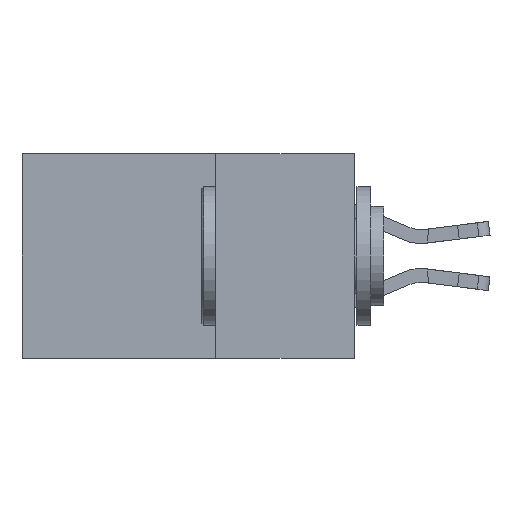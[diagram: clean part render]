
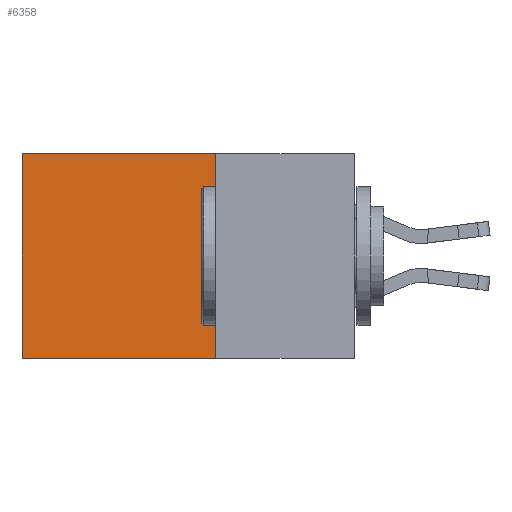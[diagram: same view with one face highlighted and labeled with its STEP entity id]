
A CAD part, left-side view. The second image highlights one B-rep face of the part: STEP entity #6358.
In plain terms, the highlighted planar face has unit normal (-1, 0, 0).
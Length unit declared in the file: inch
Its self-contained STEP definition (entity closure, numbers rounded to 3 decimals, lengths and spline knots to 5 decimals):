
#101 = LINE ( 'NONE', #17166, #5047 ) ;
#1664 = VECTOR ( 'NONE', #15389, 39.37008 ) ;
#1734 = VERTEX_POINT ( 'NONE', #1773 ) ;
#1773 = CARTESIAN_POINT ( 'NONE',  ( 0.298, 0.6, 0. ) ) ;
#2324 = EDGE_CURVE ( 'NONE', #1734, #3063, #101, .T. ) ;
#2328 = LINE ( 'NONE', #13277, #1664 ) ;
#3034 = VECTOR ( 'NONE', #15532, 39.37008 ) ;
#3063 = VERTEX_POINT ( 'NONE', #16732 ) ;
#3179 = ORIENTED_EDGE ( 'NONE', *, *, #2324, .T. ) ;
#3963 = EDGE_CURVE ( 'NONE', #17649, #3063, #8640, .T. ) ;
#4209 = CARTESIAN_POINT ( 'NONE',  ( 0.298, 0.25, 0. ) ) ;
#5047 = VECTOR ( 'NONE', #17201, 39.37008 ) ;
#6358 = ADVANCED_FACE ( 'NONE', ( #7459 ), #25138, .F. ) ;
#7459 = FACE_OUTER_BOUND ( 'NONE', #21451, .T. ) ;
#7604 = AXIS2_PLACEMENT_3D ( 'NONE', #24781, #22702, #22468 ) ;
#8640 = LINE ( 'NONE', #18347, #3034 ) ;
#8974 = CARTESIAN_POINT ( 'NONE',  ( 0.298, 0.25, -0.37 ) ) ;
#13277 = CARTESIAN_POINT ( 'NONE',  ( 0.298, 0.25, 0. ) ) ;
#13400 = DIRECTION ( 'NONE',  ( 0., 1., 0. ) ) ;
#14875 = EDGE_CURVE ( 'NONE', #24538, #1734, #20680, .T. ) ;
#15134 = VECTOR ( 'NONE', #13400, 39.37008 ) ;
#15389 = DIRECTION ( 'NONE',  ( 0., 0., -1. ) ) ;
#15532 = DIRECTION ( 'NONE',  ( 0., 1., 0. ) ) ;
#16732 = CARTESIAN_POINT ( 'NONE',  ( 0.298, 0.6, -0.37 ) ) ;
#17166 = CARTESIAN_POINT ( 'NONE',  ( 0.298, 0.6, 0. ) ) ;
#17201 = DIRECTION ( 'NONE',  ( 0., 0., -1. ) ) ;
#17649 = VERTEX_POINT ( 'NONE', #8974 ) ;
#18010 = ORIENTED_EDGE ( 'NONE', *, *, #18244, .F. ) ;
#18244 = EDGE_CURVE ( 'NONE', #24538, #17649, #2328, .T. ) ;
#18347 = CARTESIAN_POINT ( 'NONE',  ( 0.298, 0.25, -0.37 ) ) ;
#20680 = LINE ( 'NONE', #25838, #15134 ) ;
#21451 = EDGE_LOOP ( 'NONE', ( #3179, #27004, #18010, #24605 ) ) ;
#22468 = DIRECTION ( 'NONE',  ( 0., 0., -1. ) ) ;
#22702 = DIRECTION ( 'NONE',  ( 1., 0., 0. ) ) ;
#24538 = VERTEX_POINT ( 'NONE', #4209 ) ;
#24605 = ORIENTED_EDGE ( 'NONE', *, *, #14875, .T. ) ;
#24781 = CARTESIAN_POINT ( 'NONE',  ( 0.298, 0.25, 0. ) ) ;
#25138 = PLANE ( 'NONE',  #7604 ) ;
#25838 = CARTESIAN_POINT ( 'NONE',  ( 0.298, 0.25, 0. ) ) ;
#27004 = ORIENTED_EDGE ( 'NONE', *, *, #3963, .F. ) ;
